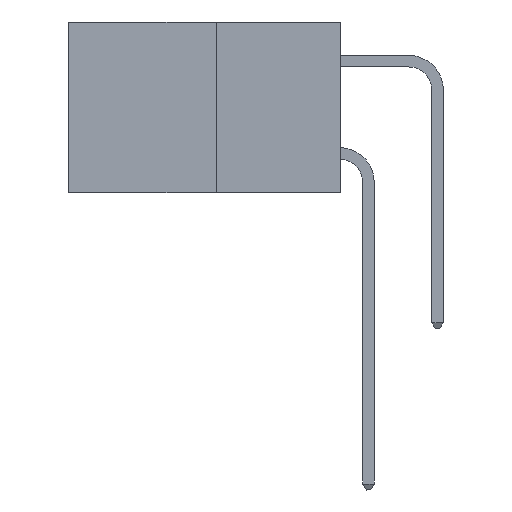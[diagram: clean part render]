
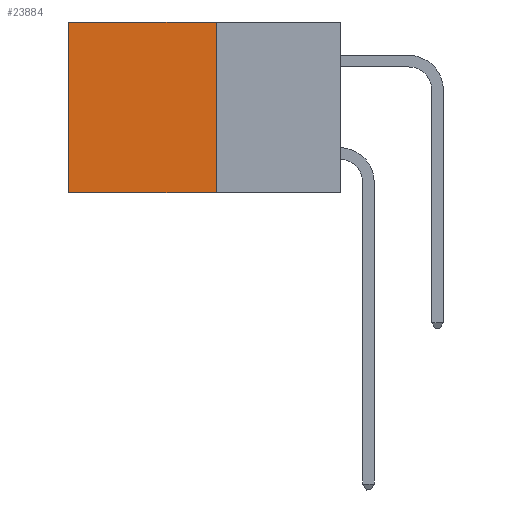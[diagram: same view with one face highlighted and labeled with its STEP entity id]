
A CAD part, left-side view. The second image highlights one B-rep face of the part: STEP entity #23884.
In plain terms, the highlighted planar face has unit normal (-1, 0, 0).
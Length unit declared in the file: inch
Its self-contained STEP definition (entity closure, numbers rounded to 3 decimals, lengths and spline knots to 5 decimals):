
#1318 = CARTESIAN_POINT ( 'NONE',  ( 0.277, 0.27, -0.37 ) ) ;
#2457 = CARTESIAN_POINT ( 'NONE',  ( 0.277, 0.27, 0. ) ) ;
#3365 = VERTEX_POINT ( 'NONE', #29802 ) ;
#3834 = EDGE_CURVE ( 'NONE', #3365, #17557, #16916, .T. ) ;
#5478 = VERTEX_POINT ( 'NONE', #31954 ) ;
#6194 = EDGE_CURVE ( 'NONE', #26348, #5478, #20102, .T. ) ;
#6269 = VECTOR ( 'NONE', #18344, 39.37008 ) ;
#6571 = DIRECTION ( 'NONE',  ( 0., 0., -1. ) ) ;
#7066 = CARTESIAN_POINT ( 'NONE',  ( 0.277, 0.27, -0.37 ) ) ;
#7074 = LINE ( 'NONE', #7066, #13245 ) ;
#7234 = CARTESIAN_POINT ( 'NONE',  ( 0.277, 0.59, -0.37 ) ) ;
#7650 = DIRECTION ( 'NONE',  ( 0., 0., -1. ) ) ;
#7795 = CARTESIAN_POINT ( 'NONE',  ( 0.277, 0.59, -0.37 ) ) ;
#10821 = FACE_OUTER_BOUND ( 'NONE', #19137, .T. ) ;
#10892 = VECTOR ( 'NONE', #7650, 39.37008 ) ;
#12860 = VECTOR ( 'NONE', #25906, 39.37008 ) ;
#13245 = VECTOR ( 'NONE', #32787, 39.37008 ) ;
#15592 = CARTESIAN_POINT ( 'NONE',  ( 0.277, 0.27, 0. ) ) ;
#16397 = EDGE_CURVE ( 'NONE', #26348, #3365, #19708, .T. ) ;
#16916 = LINE ( 'NONE', #7795, #10892 ) ;
#17557 = VERTEX_POINT ( 'NONE', #7234 ) ;
#18261 = EDGE_CURVE ( 'NONE', #5478, #17557, #7074, .T. ) ;
#18344 = DIRECTION ( 'NONE',  ( 0., 0., -1. ) ) ;
#18493 = CARTESIAN_POINT ( 'NONE',  ( 0.277, 0.27, -0.37 ) ) ;
#19137 = EDGE_LOOP ( 'NONE', ( #29847, #24332, #19324, #26064 ) ) ;
#19324 = ORIENTED_EDGE ( 'NONE', *, *, #6194, .F. ) ;
#19529 = PLANE ( 'NONE',  #31274 ) ;
#19708 = LINE ( 'NONE', #15592, #12860 ) ;
#20102 = LINE ( 'NONE', #18493, #6269 ) ;
#22054 = DIRECTION ( 'NONE',  ( 1., 0., 0. ) ) ;
#23884 = ADVANCED_FACE ( 'NONE', ( #10821 ), #19529, .F. ) ;
#24332 = ORIENTED_EDGE ( 'NONE', *, *, #18261, .F. ) ;
#25906 = DIRECTION ( 'NONE',  ( 0., 1., 0. ) ) ;
#26064 = ORIENTED_EDGE ( 'NONE', *, *, #16397, .T. ) ;
#26348 = VERTEX_POINT ( 'NONE', #2457 ) ;
#29802 = CARTESIAN_POINT ( 'NONE',  ( 0.277, 0.59, 0. ) ) ;
#29847 = ORIENTED_EDGE ( 'NONE', *, *, #3834, .T. ) ;
#31274 = AXIS2_PLACEMENT_3D ( 'NONE', #1318, #22054, #6571 ) ;
#31954 = CARTESIAN_POINT ( 'NONE',  ( 0.277, 0.27, -0.37 ) ) ;
#32787 = DIRECTION ( 'NONE',  ( 0., 1., 0. ) ) ;
